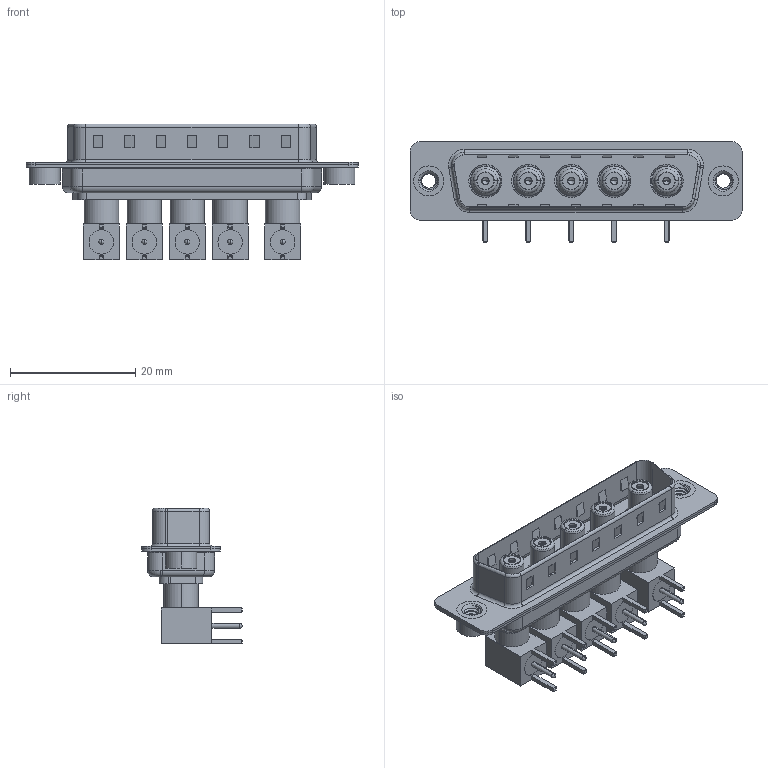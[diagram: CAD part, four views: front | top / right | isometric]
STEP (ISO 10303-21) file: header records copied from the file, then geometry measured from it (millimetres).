
FILE_DESCRIPTION (( 'STEP AP203' ), '1' );
FILE_NAME ('629-5W5-240-7NA.STEP', '2022-05-07T06:10:45', ( '' ), ( '' ), 'SwSTEP 2.0', 'SolidWorks 2020', '' );
FILE_SCHEMA (( 'CONFIG_CONTROL_DESIGN' ));
Length unit declared in the file: millimetre
Products named in the file (17): Co-Ax Jack_RA PC Tail; Socket_RA; Co-Ax Jack Assy_RA; 629Combo Threaded Rivet_2; 629Combo Shell Rear_25 Contacts; RA Back Shell; Locking Collar; 629-5W5-240-7NA; Insulator Socket; 629Combo Shell Front_25 Contacts; Insulator RA Pin; Insulator Socket 2; 629Combo Housing_5W5
Assembly tree (45 placements, depth 3):
  629-5W5-240-7NA
    629Combo Housing_5W5
    629Combo Shell Rear_25 Contacts
    629Combo Shell Front_25 Contacts
    629Combo Threaded Rivet_2  x2
    Co-Ax Jack Assy_RA
      Co-Ax Jack_RA PC Tail
      Insulator Socket
      Insulator Socket 2
      Locking Collar
      Socket_RA
      RA Back Shell
      Insulator RA Pin
    Co-Ax Jack Assy_RA
      Co-Ax Jack_RA PC Tail
      Insulator Socket
      Insulator Socket 2
      Locking Collar
      Socket_RA
      RA Back Shell
      Insulator RA Pin
    Co-Ax Jack Assy_RA
      Co-Ax Jack_RA PC Tail
      Insulator Socket
      Insulator Socket 2
      Locking Collar
      Socket_RA
      RA Back Shell
      Insulator RA Pin
    Co-Ax Jack Assy_RA
      Co-Ax Jack_RA PC Tail
      Insulator Socket
      Insulator Socket 2
      Locking Collar
      Socket_RA
      RA Back Shell
      Insulator RA Pin
    Co-Ax Jack Assy_RA
      Co-Ax Jack_RA PC Tail
      Insulator Socket
      Insulator Socket 2
      Locking Collar
      Socket_RA
      RA Back Shell
      Insulator RA Pin
Bounding box: 53.05 x 16 x 21.71 mm (x, y, z)
Volume: 4144.5 mm3; surface area: 11369 mm2
Topology: 40 solids, 40 shells, 1136 faces, 2682 edges, 1667 vertices
Faces by surface type: cylinder 472, plane 456, cone 107, torus 80, bspline 11, sphere 10
Entity records: 19562 total; most frequent: CARTESIAN_POINT 4350, DIRECTION 2802, ORIENTED_EDGE 2514, EDGE_CURVE 1257, AXIS2_PLACEMENT_3D 1046, VERTEX_POINT 793, LINE 710, VECTOR 710
